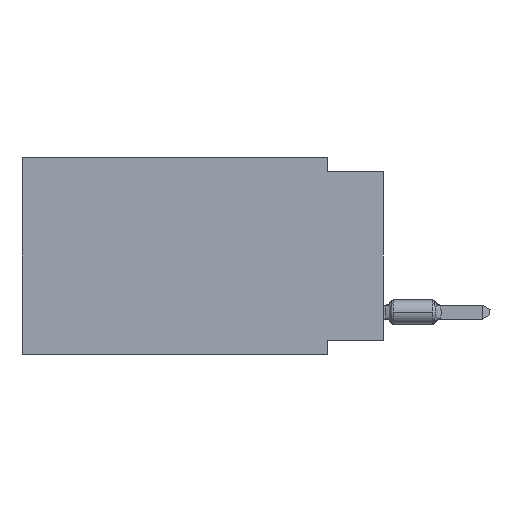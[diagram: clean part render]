
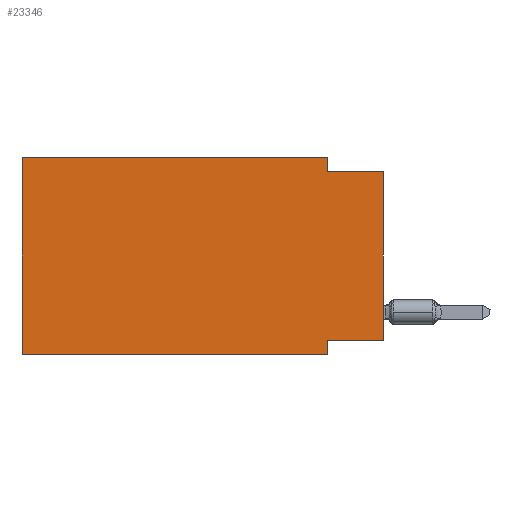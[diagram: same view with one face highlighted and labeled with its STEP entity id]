
A CAD part, left-side view. The second image highlights one B-rep face of the part: STEP entity #23346.
In plain terms, the highlighted planar face has unit normal (-1, 0, 0).
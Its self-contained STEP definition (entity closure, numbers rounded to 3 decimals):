
#272 = VECTOR ( 'NONE', #18381, 1000. ) ;
#285 = CARTESIAN_POINT ( 'NONE',  ( 0., 2.54, -8.255 ) ) ;
#333 = DIRECTION ( 'NONE',  ( 0., 0., 1. ) ) ;
#599 = LINE ( 'NONE', #22949, #16287 ) ;
#1031 = CARTESIAN_POINT ( 'NONE',  ( 0., 16.383, 0. ) ) ;
#1109 = VERTEX_POINT ( 'NONE', #285 ) ;
#1165 = FACE_OUTER_BOUND ( 'NONE', #17181, .T. ) ;
#1292 = CARTESIAN_POINT ( 'NONE',  ( 0., 2.54, 0. ) ) ;
#2017 = VECTOR ( 'NONE', #19204, 1000. ) ;
#2099 = LINE ( 'NONE', #13283, #14971 ) ;
#2307 = EDGE_CURVE ( 'NONE', #17056, #1109, #13543, .T. ) ;
#2345 = DIRECTION ( 'NONE',  ( 0., 0., -1. ) ) ;
#2516 = DIRECTION ( 'NONE',  ( 0., 0., 1. ) ) ;
#2586 = CARTESIAN_POINT ( 'NONE',  ( 0., 0., -8.255 ) ) ;
#2660 = EDGE_CURVE ( 'NONE', #1109, #21242, #2099, .T. ) ;
#3287 = ORIENTED_EDGE ( 'NONE', *, *, #23551, .F. ) ;
#3831 = VERTEX_POINT ( 'NONE', #12207 ) ;
#5796 = EDGE_CURVE ( 'NONE', #19166, #22688, #20847, .T. ) ;
#5843 = LINE ( 'NONE', #13343, #19962 ) ;
#6003 = DIRECTION ( 'NONE',  ( 0., -1., 0. ) ) ;
#6032 = ORIENTED_EDGE ( 'NONE', *, *, #23391, .F. ) ;
#6222 = CARTESIAN_POINT ( 'NONE',  ( 0., 16.383, -8.89 ) ) ;
#6573 = EDGE_CURVE ( 'NONE', #16597, #12805, #599, .T. ) ;
#6720 = CARTESIAN_POINT ( 'NONE',  ( 0., 16.383, -8.89 ) ) ;
#7295 = DIRECTION ( 'NONE',  ( 0., -1., 0. ) ) ;
#7413 = ORIENTED_EDGE ( 'NONE', *, *, #12853, .T. ) ;
#7752 = LINE ( 'NONE', #6720, #24270 ) ;
#8379 = CARTESIAN_POINT ( 'NONE',  ( 0., 16.383, 0. ) ) ;
#8392 = VECTOR ( 'NONE', #333, 1000. ) ;
#8532 = DIRECTION ( 'NONE',  ( 0., 0., -1. ) ) ;
#9879 = ORIENTED_EDGE ( 'NONE', *, *, #2660, .F. ) ;
#10737 = CARTESIAN_POINT ( 'NONE',  ( 0., 2.54, -0.635 ) ) ;
#10746 = PLANE ( 'NONE',  #10857 ) ;
#10857 = AXIS2_PLACEMENT_3D ( 'NONE', #1031, #19834, #8532 ) ;
#11944 = ORIENTED_EDGE ( 'NONE', *, *, #6573, .F. ) ;
#12207 = CARTESIAN_POINT ( 'NONE',  ( 0., 2.54, 0. ) ) ;
#12805 = VERTEX_POINT ( 'NONE', #20659 ) ;
#12853 = EDGE_CURVE ( 'NONE', #19166, #21242, #7752, .T. ) ;
#13087 = CARTESIAN_POINT ( 'NONE',  ( 0., 16.383, 0. ) ) ;
#13194 = LINE ( 'NONE', #13087, #22264 ) ;
#13283 = CARTESIAN_POINT ( 'NONE',  ( 0., 2.54, -8.89 ) ) ;
#13343 = CARTESIAN_POINT ( 'NONE',  ( 0., 0., 0. ) ) ;
#13543 = LINE ( 'NONE', #20921, #2017 ) ;
#13990 = CARTESIAN_POINT ( 'NONE',  ( 0., 2.54, -8.89 ) ) ;
#14971 = VECTOR ( 'NONE', #2345, 1000. ) ;
#16287 = VECTOR ( 'NONE', #6003, 1000. ) ;
#16597 = VERTEX_POINT ( 'NONE', #10737 ) ;
#16899 = ORIENTED_EDGE ( 'NONE', *, *, #5796, .F. ) ;
#17056 = VERTEX_POINT ( 'NONE', #2586 ) ;
#17164 = CARTESIAN_POINT ( 'NONE',  ( 0., 16.383, 0. ) ) ;
#17181 = EDGE_LOOP ( 'NONE', ( #20560, #11944, #6032, #3287, #16899, #7413, #9879, #22908 ) ) ;
#18381 = DIRECTION ( 'NONE',  ( 0., 0., -1. ) ) ;
#19166 = VERTEX_POINT ( 'NONE', #6222 ) ;
#19204 = DIRECTION ( 'NONE',  ( 0., 1., 0. ) ) ;
#19305 = DIRECTION ( 'NONE',  ( 0., -1., 0. ) ) ;
#19834 = DIRECTION ( 'NONE',  ( 1., 0., 0. ) ) ;
#19962 = VECTOR ( 'NONE', #2516, 1000. ) ;
#20560 = ORIENTED_EDGE ( 'NONE', *, *, #22029, .T. ) ;
#20659 = CARTESIAN_POINT ( 'NONE',  ( 0., 0., -0.635 ) ) ;
#20847 = LINE ( 'NONE', #17164, #8392 ) ;
#20921 = CARTESIAN_POINT ( 'NONE',  ( 0., 0., -8.255 ) ) ;
#21242 = VERTEX_POINT ( 'NONE', #13990 ) ;
#21675 = LINE ( 'NONE', #1292, #272 ) ;
#22029 = EDGE_CURVE ( 'NONE', #17056, #12805, #5843, .T. ) ;
#22264 = VECTOR ( 'NONE', #7295, 1000. ) ;
#22688 = VERTEX_POINT ( 'NONE', #8379 ) ;
#22908 = ORIENTED_EDGE ( 'NONE', *, *, #2307, .F. ) ;
#22949 = CARTESIAN_POINT ( 'NONE',  ( 0., 0., -0.635 ) ) ;
#23346 = ADVANCED_FACE ( 'NONE', ( #1165 ), #10746, .F. ) ;
#23391 = EDGE_CURVE ( 'NONE', #3831, #16597, #21675, .T. ) ;
#23551 = EDGE_CURVE ( 'NONE', #22688, #3831, #13194, .T. ) ;
#24270 = VECTOR ( 'NONE', #19305, 1000. ) ;
